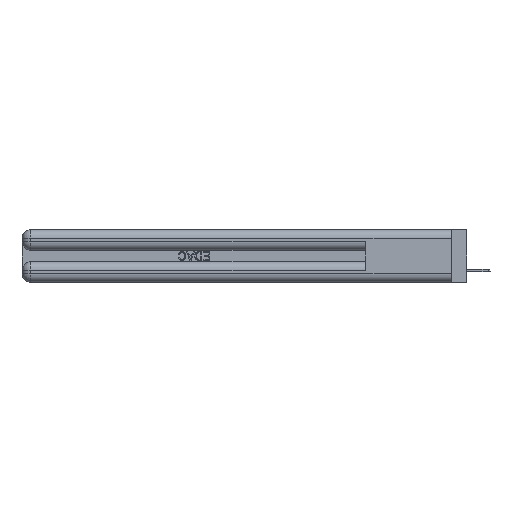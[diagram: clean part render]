
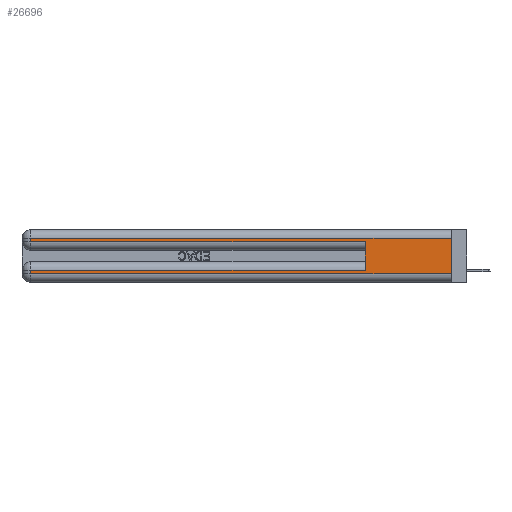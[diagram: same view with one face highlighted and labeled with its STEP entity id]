
A CAD part, left-side view. The second image highlights one B-rep face of the part: STEP entity #26696.
In plain terms, the highlighted planar face has unit normal (-1, 0, 0).
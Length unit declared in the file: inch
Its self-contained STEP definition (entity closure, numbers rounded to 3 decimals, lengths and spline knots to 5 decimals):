
#117 = VECTOR ( 'NONE', #36425, 39.37008 ) ;
#712 = CARTESIAN_POINT ( 'NONE',  ( 0., 2.94, 0.085 ) ) ;
#992 = EDGE_CURVE ( 'NONE', #5402, #9099, #21316, .T. ) ;
#1303 = ORIENTED_EDGE ( 'NONE', *, *, #30049, .T. ) ;
#1351 = CARTESIAN_POINT ( 'NONE',  ( 0., 2.94, 0.37 ) ) ;
#2123 = PLANE ( 'NONE',  #32181 ) ;
#2241 = DIRECTION ( 'NONE',  ( 0., 0., -1. ) ) ;
#2670 = LINE ( 'NONE', #25320, #14753 ) ;
#3237 = VERTEX_POINT ( 'NONE', #30917 ) ;
#3787 = DIRECTION ( 'NONE',  ( 0., 0., -1. ) ) ;
#3797 = LINE ( 'NONE', #35908, #28766 ) ;
#4183 = VECTOR ( 'NONE', #30777, 39.37008 ) ;
#4915 = DIRECTION ( 'NONE',  ( 0., 1., 0. ) ) ;
#5402 = VERTEX_POINT ( 'NONE', #31200 ) ;
#6311 = CARTESIAN_POINT ( 'NONE',  ( 0., 2.94, 0.06 ) ) ;
#6399 = VERTEX_POINT ( 'NONE', #712 ) ;
#6420 = VECTOR ( 'NONE', #13244, 39.37008 ) ;
#6568 = CARTESIAN_POINT ( 'NONE',  ( 0., 0., 0.31 ) ) ;
#7306 = VERTEX_POINT ( 'NONE', #15674 ) ;
#8166 = CARTESIAN_POINT ( 'NONE',  ( 0., 0., 0.37 ) ) ;
#8325 = LINE ( 'NONE', #33709, #6420 ) ;
#8380 = VERTEX_POINT ( 'NONE', #6568 ) ;
#9099 = VERTEX_POINT ( 'NONE', #10529 ) ;
#10529 = CARTESIAN_POINT ( 'NONE',  ( 0., 2.94, 0.285 ) ) ;
#10555 = EDGE_CURVE ( 'NONE', #13798, #3237, #8325, .T. ) ;
#10824 = EDGE_CURVE ( 'NONE', #8380, #5402, #17158, .T. ) ;
#13244 = DIRECTION ( 'NONE',  ( 0., 0., 1. ) ) ;
#13706 = CARTESIAN_POINT ( 'NONE',  ( 0., 0.6, 0.085 ) ) ;
#13798 = VERTEX_POINT ( 'NONE', #13706 ) ;
#14753 = VECTOR ( 'NONE', #24951, 39.37008 ) ;
#15674 = CARTESIAN_POINT ( 'NONE',  ( 0., 0., 0.06 ) ) ;
#15744 = ORIENTED_EDGE ( 'NONE', *, *, #10555, .F. ) ;
#16071 = EDGE_CURVE ( 'NONE', #6399, #38125, #31937, .T. ) ;
#17158 = LINE ( 'NONE', #37277, #25395 ) ;
#17620 = CARTESIAN_POINT ( 'NONE',  ( 0., 2.94, 0.37 ) ) ;
#18684 = LINE ( 'NONE', #30638, #117 ) ;
#20686 = ORIENTED_EDGE ( 'NONE', *, *, #10824, .T. ) ;
#20904 = LINE ( 'NONE', #28932, #32409 ) ;
#21316 = LINE ( 'NONE', #1351, #4183 ) ;
#21376 = ORIENTED_EDGE ( 'NONE', *, *, #36198, .F. ) ;
#21884 = ORIENTED_EDGE ( 'NONE', *, *, #22024, .T. ) ;
#22024 = EDGE_CURVE ( 'NONE', #38125, #7306, #2670, .T. ) ;
#24109 = DIRECTION ( 'NONE',  ( 0., -1., 0. ) ) ;
#24951 = DIRECTION ( 'NONE',  ( 0., -1., 0. ) ) ;
#25320 = CARTESIAN_POINT ( 'NONE',  ( 0., 0., 0.06 ) ) ;
#25395 = VECTOR ( 'NONE', #4915, 39.37008 ) ;
#25449 = ORIENTED_EDGE ( 'NONE', *, *, #992, .T. ) ;
#26696 = ADVANCED_FACE ( 'NONE', ( #29542 ), #2123, .F. ) ;
#27879 = ORIENTED_EDGE ( 'NONE', *, *, #16071, .T. ) ;
#28766 = VECTOR ( 'NONE', #24109, 39.37008 ) ;
#28932 = CARTESIAN_POINT ( 'NONE',  ( 0., 0., 0.085 ) ) ;
#29542 = FACE_OUTER_BOUND ( 'NONE', #31407, .T. ) ;
#30049 = EDGE_CURVE ( 'NONE', #9099, #3237, #3797, .T. ) ;
#30638 = CARTESIAN_POINT ( 'NONE',  ( 0., 0., 0.37 ) ) ;
#30777 = DIRECTION ( 'NONE',  ( 0., 0., -1. ) ) ;
#30917 = CARTESIAN_POINT ( 'NONE',  ( 0., 0.6, 0.285 ) ) ;
#31200 = CARTESIAN_POINT ( 'NONE',  ( 0., 2.94, 0.31 ) ) ;
#31407 = EDGE_LOOP ( 'NONE', ( #21376, #20686, #25449, #1303, #15744, #38106, #27879, #21884 ) ) ;
#31531 = DIRECTION ( 'NONE',  ( 1., 0., 0. ) ) ;
#31937 = LINE ( 'NONE', #17620, #37699 ) ;
#32181 = AXIS2_PLACEMENT_3D ( 'NONE', #8166, #31531, #2241 ) ;
#32263 = DIRECTION ( 'NONE',  ( 0., 1., 0. ) ) ;
#32409 = VECTOR ( 'NONE', #32263, 39.37008 ) ;
#33709 = CARTESIAN_POINT ( 'NONE',  ( 0., 0.6, 0.145 ) ) ;
#35908 = CARTESIAN_POINT ( 'NONE',  ( 0., 0., 0.285 ) ) ;
#36198 = EDGE_CURVE ( 'NONE', #8380, #7306, #18684, .T. ) ;
#36425 = DIRECTION ( 'NONE',  ( 0., 0., -1. ) ) ;
#37277 = CARTESIAN_POINT ( 'NONE',  ( 0., 0., 0.31 ) ) ;
#37311 = EDGE_CURVE ( 'NONE', #13798, #6399, #20904, .T. ) ;
#37699 = VECTOR ( 'NONE', #3787, 39.37008 ) ;
#38106 = ORIENTED_EDGE ( 'NONE', *, *, #37311, .T. ) ;
#38125 = VERTEX_POINT ( 'NONE', #6311 ) ;
